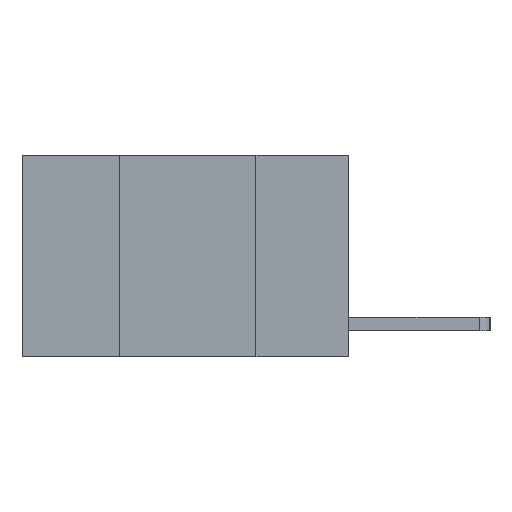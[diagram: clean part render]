
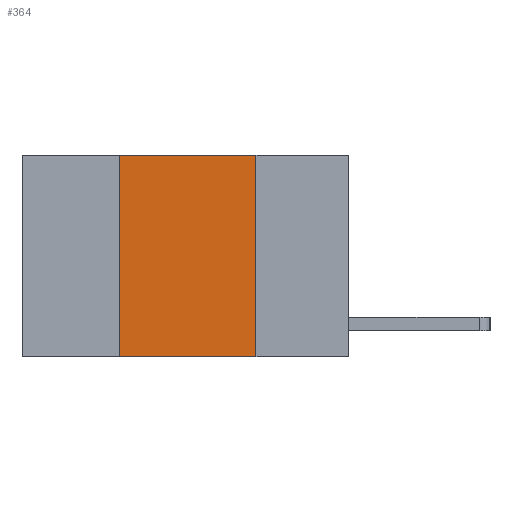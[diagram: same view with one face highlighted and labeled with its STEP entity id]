
A CAD part, left-side view. The second image highlights one B-rep face of the part: STEP entity #364.
In plain terms, the highlighted planar face has unit normal (-1, 0, 0).
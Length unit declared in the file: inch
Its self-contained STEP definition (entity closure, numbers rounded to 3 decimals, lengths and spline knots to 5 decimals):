
#42 = EDGE_CURVE ( 'NONE', #4887, #8520, #8725, .T. ) ;
#114 = CARTESIAN_POINT ( 'NONE',  ( 0., 0.17, 0. ) ) ;
#364 = ADVANCED_FACE ( 'NONE', ( #8800 ), #8387, .F. ) ;
#386 = DIRECTION ( 'NONE',  ( 0., 0., 1. ) ) ;
#572 = VECTOR ( 'NONE', #3463, 39.37008 ) ;
#711 = CARTESIAN_POINT ( 'NONE',  ( 0., 0.17, -0.37 ) ) ;
#733 = ORIENTED_EDGE ( 'NONE', *, *, #2824, .T. ) ;
#1333 = EDGE_LOOP ( 'NONE', ( #5815, #6652, #6933, #733 ) ) ;
#1749 = DIRECTION ( 'NONE',  ( 0., 0., -1. ) ) ;
#2019 = LINE ( 'NONE', #5614, #572 ) ;
#2081 = VERTEX_POINT ( 'NONE', #5779 ) ;
#2235 = AXIS2_PLACEMENT_3D ( 'NONE', #9005, #7744, #7996 ) ;
#2301 = EDGE_CURVE ( 'NONE', #8520, #2081, #2019, .T. ) ;
#2824 = EDGE_CURVE ( 'NONE', #4887, #9125, #3150, .T. ) ;
#3150 = LINE ( 'NONE', #8183, #4832 ) ;
#3250 = VECTOR ( 'NONE', #1749, 39.37008 ) ;
#3463 = DIRECTION ( 'NONE',  ( 0., -1., 0. ) ) ;
#3588 = EDGE_CURVE ( 'NONE', #2081, #9125, #5149, .T. ) ;
#4444 = CARTESIAN_POINT ( 'NONE',  ( 0., 0.42, -0.37 ) ) ;
#4816 = CARTESIAN_POINT ( 'NONE',  ( 0., 0.42, 0. ) ) ;
#4832 = VECTOR ( 'NONE', #7849, 39.37008 ) ;
#4887 = VERTEX_POINT ( 'NONE', #4444 ) ;
#5149 = LINE ( 'NONE', #114, #3250 ) ;
#5614 = CARTESIAN_POINT ( 'NONE',  ( 0., 0.6, 0. ) ) ;
#5779 = CARTESIAN_POINT ( 'NONE',  ( 0., 0.17, 0. ) ) ;
#5815 = ORIENTED_EDGE ( 'NONE', *, *, #3588, .F. ) ;
#6652 = ORIENTED_EDGE ( 'NONE', *, *, #2301, .F. ) ;
#6933 = ORIENTED_EDGE ( 'NONE', *, *, #42, .F. ) ;
#7744 = DIRECTION ( 'NONE',  ( 1., 0., 0. ) ) ;
#7849 = DIRECTION ( 'NONE',  ( 0., -1., 0. ) ) ;
#7996 = DIRECTION ( 'NONE',  ( 0., 0., -1. ) ) ;
#8183 = CARTESIAN_POINT ( 'NONE',  ( 0., 0.6, -0.37 ) ) ;
#8300 = VECTOR ( 'NONE', #386, 39.37008 ) ;
#8387 = PLANE ( 'NONE',  #2235 ) ;
#8485 = CARTESIAN_POINT ( 'NONE',  ( 0., 0.42, 0. ) ) ;
#8520 = VERTEX_POINT ( 'NONE', #8485 ) ;
#8725 = LINE ( 'NONE', #4816, #8300 ) ;
#8800 = FACE_OUTER_BOUND ( 'NONE', #1333, .T. ) ;
#9005 = CARTESIAN_POINT ( 'NONE',  ( 0., 0.6, 0. ) ) ;
#9125 = VERTEX_POINT ( 'NONE', #711 ) ;
